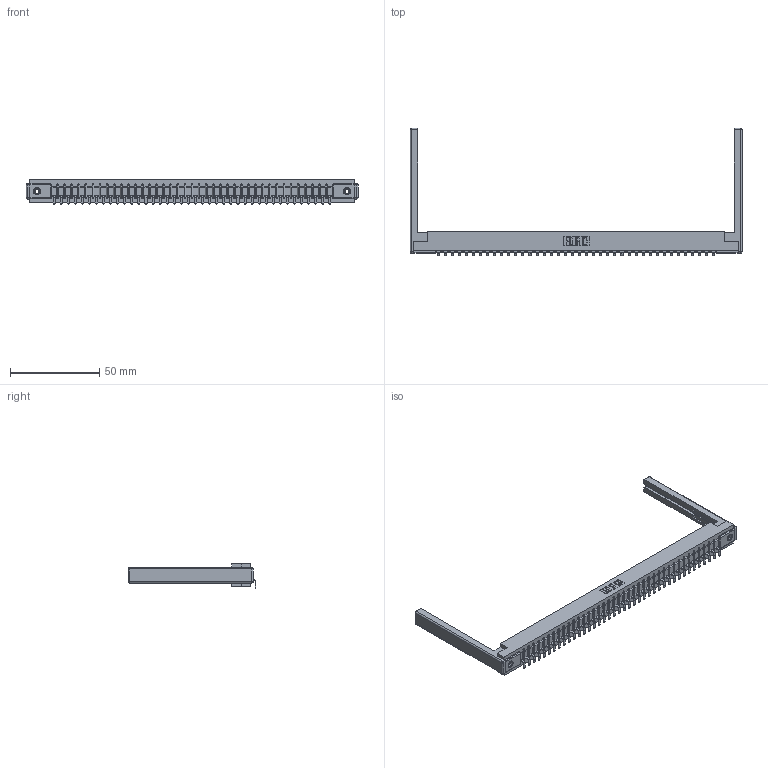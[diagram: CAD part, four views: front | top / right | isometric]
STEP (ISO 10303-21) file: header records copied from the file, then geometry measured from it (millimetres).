
FILE_DESCRIPTION (( 'STEP AP203' ), '1' );
FILE_NAME ('357-040-553-168.STEP', '2019-09-17T09:12:35', ( '' ), ( '' ), 'SwSTEP 2.0', 'SolidWorks 2016', '' );
FILE_SCHEMA (( 'CONFIG_CONTROL_DESIGN' ));
Length unit declared in the file: inch
Products named in the file (5): 307 Part_.156 Dia Mounting Holes; 357-040-553-168; 307-290-002_553; 345-250-001_345-250-001-102; 307-220-068
Assembly tree (45 placements, depth 2):
  357-040-553-168
    307 Part_.156 Dia Mounting Holes
    307-290-002_553  x40
    307-220-068  x2
    345-250-001_345-250-001-102  x2
Bounding box: 185.93 x 71.29 x 13.5 mm (x, y, z)
Volume: 24259.2 mm3; surface area: 28908.9 mm2
Topology: 45 solids, 45 shells, 3433 faces, 10473 edges, 6850 vertices
Faces by surface type: plane 2038, cylinder 1289, sphere 90, cone 12, torus 4
Entity records: 38151 total; most frequent: CARTESIAN_POINT 6401, ORIENTED_EDGE 6380, DIRECTION 6238, EDGE_CURVE 3190, VECTOR 2440, LINE 2440, VERTEX_POINT 2062, AXIS2_PLACEMENT_3D 1899
